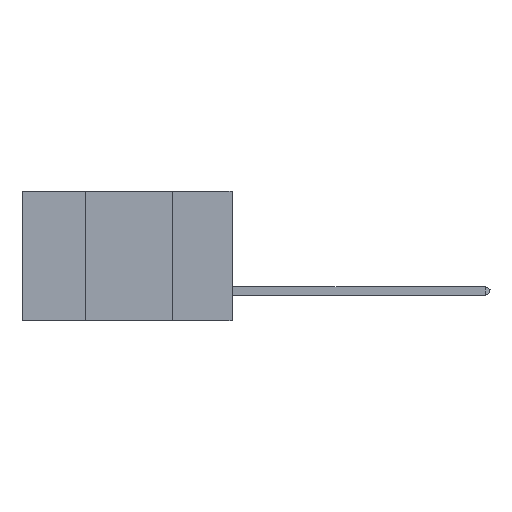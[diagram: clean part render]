
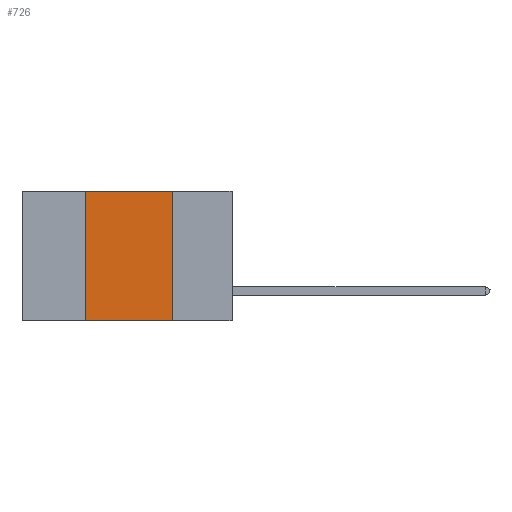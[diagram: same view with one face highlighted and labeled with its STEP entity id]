
A CAD part, left-side view. The second image highlights one B-rep face of the part: STEP entity #726.
In plain terms, the highlighted planar face has unit normal (-1, 0, 0).
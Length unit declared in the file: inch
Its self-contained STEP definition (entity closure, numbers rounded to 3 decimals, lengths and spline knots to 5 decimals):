
#554 = ORIENTED_EDGE ( 'NONE', *, *, #10132, .F. ) ;
#726 = ADVANCED_FACE ( 'NONE', ( #24377 ), #9559, .F. ) ;
#3772 = VERTEX_POINT ( 'NONE', #7107 ) ;
#3936 = ORIENTED_EDGE ( 'NONE', *, *, #16650, .F. ) ;
#4128 = ORIENTED_EDGE ( 'NONE', *, *, #13614, .T. ) ;
#4336 = CARTESIAN_POINT ( 'NONE',  ( 0., 0.6, -0.37 ) ) ;
#4530 = VECTOR ( 'NONE', #8548, 39.37008 ) ;
#5062 = LINE ( 'NONE', #20768, #10232 ) ;
#5985 = DIRECTION ( 'NONE',  ( 0., 0., -1. ) ) ;
#7107 = CARTESIAN_POINT ( 'NONE',  ( 0., 0.42, 0. ) ) ;
#7462 = CARTESIAN_POINT ( 'NONE',  ( 0., 0.6, 0. ) ) ;
#8427 = DIRECTION ( 'NONE',  ( 0., 0., 1. ) ) ;
#8548 = DIRECTION ( 'NONE',  ( 0., -1., 0. ) ) ;
#8688 = EDGE_CURVE ( 'NONE', #13820, #10264, #8995, .T. ) ;
#8995 = LINE ( 'NONE', #24183, #10004 ) ;
#9559 = PLANE ( 'NONE',  #25396 ) ;
#9826 = LINE ( 'NONE', #7462, #17281 ) ;
#10004 = VECTOR ( 'NONE', #20091, 39.37008 ) ;
#10132 = EDGE_CURVE ( 'NONE', #26180, #3772, #5062, .T. ) ;
#10232 = VECTOR ( 'NONE', #8427, 39.37008 ) ;
#10264 = VERTEX_POINT ( 'NONE', #20802 ) ;
#13614 = EDGE_CURVE ( 'NONE', #26180, #10264, #20317, .T. ) ;
#13820 = VERTEX_POINT ( 'NONE', #26048 ) ;
#16142 = DIRECTION ( 'NONE',  ( 1., 0., 0. ) ) ;
#16405 = CARTESIAN_POINT ( 'NONE',  ( 0., 0.6, 0. ) ) ;
#16456 = EDGE_LOOP ( 'NONE', ( #25759, #3936, #554, #4128 ) ) ;
#16650 = EDGE_CURVE ( 'NONE', #3772, #13820, #9826, .T. ) ;
#17281 = VECTOR ( 'NONE', #17763, 39.37008 ) ;
#17763 = DIRECTION ( 'NONE',  ( 0., -1., 0. ) ) ;
#19860 = CARTESIAN_POINT ( 'NONE',  ( 0., 0.42, -0.37 ) ) ;
#20091 = DIRECTION ( 'NONE',  ( 0., 0., -1. ) ) ;
#20317 = LINE ( 'NONE', #4336, #4530 ) ;
#20768 = CARTESIAN_POINT ( 'NONE',  ( 0., 0.42, 0. ) ) ;
#20802 = CARTESIAN_POINT ( 'NONE',  ( 0., 0.17, -0.37 ) ) ;
#24183 = CARTESIAN_POINT ( 'NONE',  ( 0., 0.17, 0. ) ) ;
#24377 = FACE_OUTER_BOUND ( 'NONE', #16456, .T. ) ;
#25396 = AXIS2_PLACEMENT_3D ( 'NONE', #16405, #16142, #5985 ) ;
#25759 = ORIENTED_EDGE ( 'NONE', *, *, #8688, .F. ) ;
#26048 = CARTESIAN_POINT ( 'NONE',  ( 0., 0.17, 0. ) ) ;
#26180 = VERTEX_POINT ( 'NONE', #19860 ) ;
